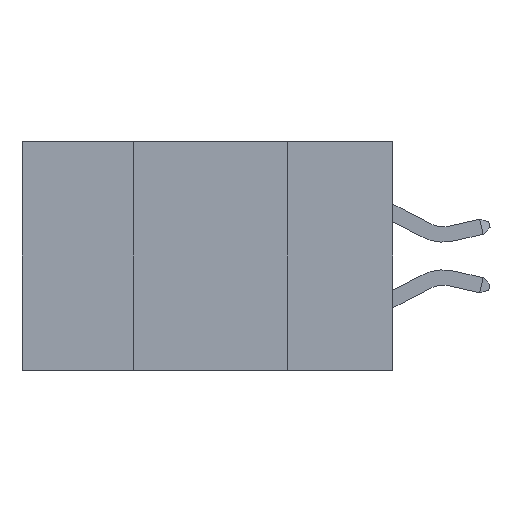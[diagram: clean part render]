
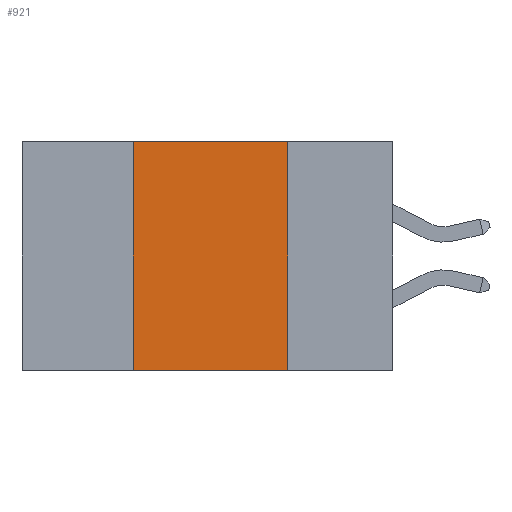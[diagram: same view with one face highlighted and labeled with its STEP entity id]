
A CAD part, left-side view. The second image highlights one B-rep face of the part: STEP entity #921.
In plain terms, the highlighted planar face has unit normal (-1, 0, 0).
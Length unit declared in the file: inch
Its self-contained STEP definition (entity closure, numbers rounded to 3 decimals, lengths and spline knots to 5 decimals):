
#642 = CARTESIAN_POINT ( 'NONE',  ( 0., 0.42, -0.37 ) ) ;
#921 = ADVANCED_FACE ( 'NONE', ( #13083 ), #4181, .F. ) ;
#1012 = VERTEX_POINT ( 'NONE', #15326 ) ;
#1856 = EDGE_LOOP ( 'NONE', ( #12399, #9489, #2144, #9892 ) ) ;
#2144 = ORIENTED_EDGE ( 'NONE', *, *, #15931, .F. ) ;
#3462 = CARTESIAN_POINT ( 'NONE',  ( 0., 0.17, -0.37 ) ) ;
#3824 = EDGE_CURVE ( 'NONE', #1012, #6104, #3970, .T. ) ;
#3970 = LINE ( 'NONE', #9907, #6963 ) ;
#4104 = VECTOR ( 'NONE', #9904, 39.37008 ) ;
#4181 = PLANE ( 'NONE',  #12798 ) ;
#4274 = VECTOR ( 'NONE', #9447, 39.37008 ) ;
#4369 = CARTESIAN_POINT ( 'NONE',  ( 0., 0.6, 0. ) ) ;
#4761 = DIRECTION ( 'NONE',  ( 1., 0., 0. ) ) ;
#5243 = DIRECTION ( 'NONE',  ( 0., 0., -1. ) ) ;
#5682 = CARTESIAN_POINT ( 'NONE',  ( 0., 0.42, 0. ) ) ;
#6104 = VERTEX_POINT ( 'NONE', #3462 ) ;
#6963 = VECTOR ( 'NONE', #14077, 39.37008 ) ;
#7321 = VERTEX_POINT ( 'NONE', #11956 ) ;
#7634 = LINE ( 'NONE', #5682, #4274 ) ;
#9429 = VECTOR ( 'NONE', #14343, 39.37008 ) ;
#9447 = DIRECTION ( 'NONE',  ( 0., 0., 1. ) ) ;
#9449 = VERTEX_POINT ( 'NONE', #642 ) ;
#9489 = ORIENTED_EDGE ( 'NONE', *, *, #11544, .F. ) ;
#9892 = ORIENTED_EDGE ( 'NONE', *, *, #15185, .T. ) ;
#9904 = DIRECTION ( 'NONE',  ( 0., -1., 0. ) ) ;
#9907 = CARTESIAN_POINT ( 'NONE',  ( 0., 0.17, 0. ) ) ;
#10408 = LINE ( 'NONE', #14670, #4104 ) ;
#11544 = EDGE_CURVE ( 'NONE', #7321, #1012, #12713, .T. ) ;
#11956 = CARTESIAN_POINT ( 'NONE',  ( 0., 0.42, 0. ) ) ;
#11985 = CARTESIAN_POINT ( 'NONE',  ( 0., 0.6, 0. ) ) ;
#12399 = ORIENTED_EDGE ( 'NONE', *, *, #3824, .F. ) ;
#12713 = LINE ( 'NONE', #11985, #9429 ) ;
#12798 = AXIS2_PLACEMENT_3D ( 'NONE', #4369, #4761, #5243 ) ;
#13083 = FACE_OUTER_BOUND ( 'NONE', #1856, .T. ) ;
#14077 = DIRECTION ( 'NONE',  ( 0., 0., -1. ) ) ;
#14343 = DIRECTION ( 'NONE',  ( 0., -1., 0. ) ) ;
#14670 = CARTESIAN_POINT ( 'NONE',  ( 0., 0.6, -0.37 ) ) ;
#15185 = EDGE_CURVE ( 'NONE', #9449, #6104, #10408, .T. ) ;
#15326 = CARTESIAN_POINT ( 'NONE',  ( 0., 0.17, 0. ) ) ;
#15931 = EDGE_CURVE ( 'NONE', #9449, #7321, #7634, .T. ) ;
